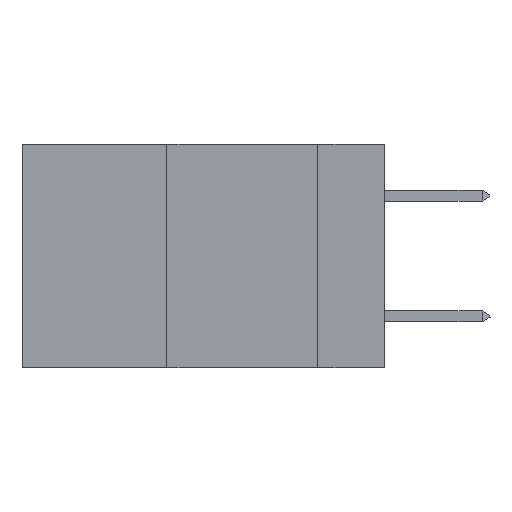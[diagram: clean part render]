
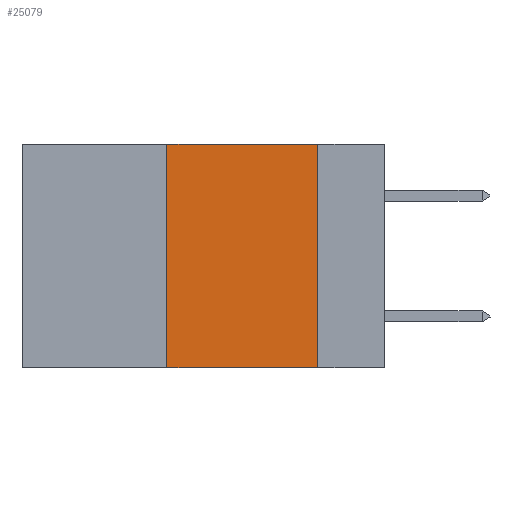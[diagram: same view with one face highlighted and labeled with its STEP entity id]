
A CAD part, left-side view. The second image highlights one B-rep face of the part: STEP entity #25079.
In plain terms, the highlighted planar face has unit normal (-1, 0, 0).
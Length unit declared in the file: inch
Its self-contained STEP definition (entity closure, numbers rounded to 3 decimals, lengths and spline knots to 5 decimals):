
#272 = LINE ( 'NONE', #5137, #8313 ) ;
#391 = ORIENTED_EDGE ( 'NONE', *, *, #37741, .F. ) ;
#1736 = ORIENTED_EDGE ( 'NONE', *, *, #44035, .T. ) ;
#2387 = CARTESIAN_POINT ( 'NONE',  ( 0., 0.6, 0. ) ) ;
#3567 = EDGE_CURVE ( 'NONE', #43818, #10476, #272, .T. ) ;
#3580 = CARTESIAN_POINT ( 'NONE',  ( 0., 0.36, -0.37 ) ) ;
#3816 = DIRECTION ( 'NONE',  ( 0., -1., 0. ) ) ;
#5137 = CARTESIAN_POINT ( 'NONE',  ( 0., 0.11, 0. ) ) ;
#6756 = VECTOR ( 'NONE', #39238, 39.37008 ) ;
#7570 = VERTEX_POINT ( 'NONE', #41180 ) ;
#8313 = VECTOR ( 'NONE', #39271, 39.37008 ) ;
#8343 = EDGE_LOOP ( 'NONE', ( #17281, #12531, #391, #1736 ) ) ;
#10476 = VERTEX_POINT ( 'NONE', #22019 ) ;
#11976 = VECTOR ( 'NONE', #3816, 39.37008 ) ;
#12448 = PLANE ( 'NONE',  #32264 ) ;
#12531 = ORIENTED_EDGE ( 'NONE', *, *, #30295, .F. ) ;
#12733 = VERTEX_POINT ( 'NONE', #3580 ) ;
#15978 = LINE ( 'NONE', #33674, #43661 ) ;
#17281 = ORIENTED_EDGE ( 'NONE', *, *, #3567, .F. ) ;
#19111 = CARTESIAN_POINT ( 'NONE',  ( 0., 0.6, -0.37 ) ) ;
#22019 = CARTESIAN_POINT ( 'NONE',  ( 0., 0.11, -0.37 ) ) ;
#25079 = ADVANCED_FACE ( 'NONE', ( #37564 ), #12448, .F. ) ;
#29200 = LINE ( 'NONE', #19111, #6756 ) ;
#30099 = CARTESIAN_POINT ( 'NONE',  ( 0., 0.6, 0. ) ) ;
#30295 = EDGE_CURVE ( 'NONE', #7570, #43818, #34345, .T. ) ;
#32264 = AXIS2_PLACEMENT_3D ( 'NONE', #2387, #36231, #32994 ) ;
#32994 = DIRECTION ( 'NONE',  ( 0., 0., -1. ) ) ;
#33674 = CARTESIAN_POINT ( 'NONE',  ( 0., 0.36, 0. ) ) ;
#34032 = CARTESIAN_POINT ( 'NONE',  ( 0., 0.11, 0. ) ) ;
#34345 = LINE ( 'NONE', #30099, #11976 ) ;
#36231 = DIRECTION ( 'NONE',  ( 1., 0., 0. ) ) ;
#37564 = FACE_OUTER_BOUND ( 'NONE', #8343, .T. ) ;
#37741 = EDGE_CURVE ( 'NONE', #12733, #7570, #15978, .T. ) ;
#39238 = DIRECTION ( 'NONE',  ( 0., -1., 0. ) ) ;
#39271 = DIRECTION ( 'NONE',  ( 0., 0., -1. ) ) ;
#40191 = DIRECTION ( 'NONE',  ( 0., 0., 1. ) ) ;
#41180 = CARTESIAN_POINT ( 'NONE',  ( 0., 0.36, 0. ) ) ;
#43661 = VECTOR ( 'NONE', #40191, 39.37008 ) ;
#43818 = VERTEX_POINT ( 'NONE', #34032 ) ;
#44035 = EDGE_CURVE ( 'NONE', #12733, #10476, #29200, .T. ) ;
